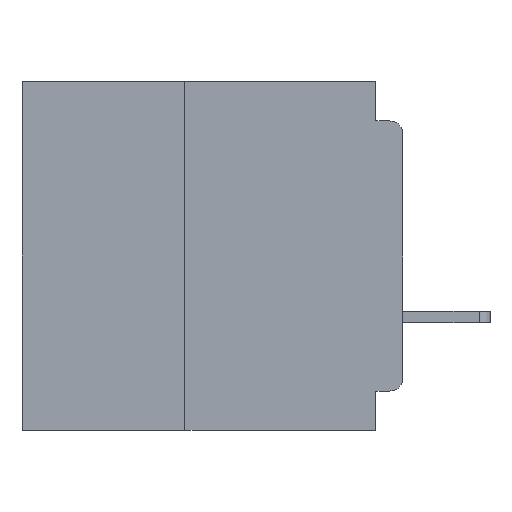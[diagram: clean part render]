
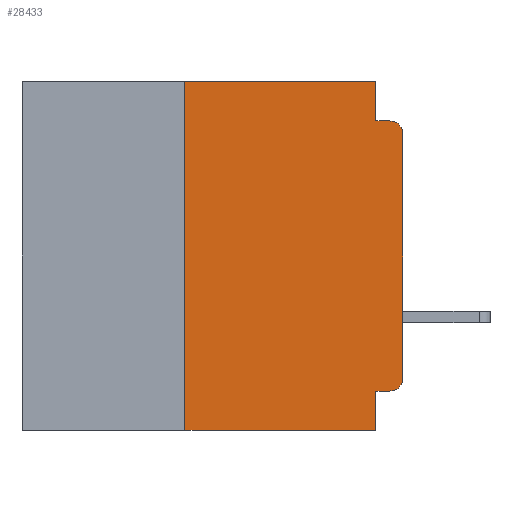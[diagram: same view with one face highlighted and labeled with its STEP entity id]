
A CAD part, left-side view. The second image highlights one B-rep face of the part: STEP entity #28433.
In plain terms, the highlighted planar face has unit normal (-1, 0, 0).
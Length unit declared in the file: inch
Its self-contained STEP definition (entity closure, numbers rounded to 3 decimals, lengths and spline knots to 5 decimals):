
#752 = CARTESIAN_POINT ( 'NONE',  ( 0., 0.031, -0.4 ) ) ;
#1406 = DIRECTION ( 'NONE',  ( 0., 0., -1. ) ) ;
#2109 = ORIENTED_EDGE ( 'NONE', *, *, #53110, .T. ) ;
#2112 = CARTESIAN_POINT ( 'NONE',  ( 0., 0.031, -0.4 ) ) ;
#2252 = FACE_OUTER_BOUND ( 'NONE', #7011, .T. ) ;
#3028 = ORIENTED_EDGE ( 'NONE', *, *, #6887, .F. ) ;
#6082 = VECTOR ( 'NONE', #15665, 39.37008 ) ;
#6200 = VECTOR ( 'NONE', #30947, 39.37008 ) ;
#6887 = EDGE_CURVE ( 'NONE', #15216, #43634, #40026, .T. ) ;
#7011 = EDGE_LOOP ( 'NONE', ( #31072, #17929, #53032, #22352, #19823, #24489, #22185, #44135, #3028, #2109 ) ) ;
#7617 = CARTESIAN_POINT ( 'NONE',  ( 0., 0.015, -0.045 ) ) ;
#7827 = CARTESIAN_POINT ( 'NONE',  ( 0., 0.25, 0. ) ) ;
#8480 = VERTEX_POINT ( 'NONE', #7617 ) ;
#9201 = CARTESIAN_POINT ( 'NONE',  ( 0., 0., 0. ) ) ;
#10609 = CARTESIAN_POINT ( 'NONE',  ( 0., 0., -0.06 ) ) ;
#11358 = CARTESIAN_POINT ( 'NONE',  ( 0., 0.437, -0.4 ) ) ;
#11630 = LINE ( 'NONE', #2112, #43968 ) ;
#11944 = CARTESIAN_POINT ( 'NONE',  ( 0., 0., -0.355 ) ) ;
#12194 = EDGE_CURVE ( 'NONE', #28208, #25364, #17548, .T. ) ;
#13304 = VECTOR ( 'NONE', #14707, 39.37008 ) ;
#13671 = EDGE_CURVE ( 'NONE', #28208, #19549, #39863, .T. ) ;
#14648 = LINE ( 'NONE', #31755, #13304 ) ;
#14707 = DIRECTION ( 'NONE',  ( 0., -1., 0. ) ) ;
#15216 = VERTEX_POINT ( 'NONE', #18132 ) ;
#15665 = DIRECTION ( 'NONE',  ( 0., -1., 0. ) ) ;
#17548 = LINE ( 'NONE', #18153, #6200 ) ;
#17929 = ORIENTED_EDGE ( 'NONE', *, *, #50631, .T. ) ;
#18132 = CARTESIAN_POINT ( 'NONE',  ( 0., 0.015, -0.355 ) ) ;
#18153 = CARTESIAN_POINT ( 'NONE',  ( 0., 0.25, -0.4 ) ) ;
#19419 = CARTESIAN_POINT ( 'NONE',  ( 0., 0.25, -0.4 ) ) ;
#19503 = VECTOR ( 'NONE', #51421, 39.37008 ) ;
#19549 = VERTEX_POINT ( 'NONE', #752 ) ;
#19823 = ORIENTED_EDGE ( 'NONE', *, *, #52072, .F. ) ;
#20182 = CARTESIAN_POINT ( 'NONE',  ( 0., 0., -0.045 ) ) ;
#20653 = DIRECTION ( 'NONE',  ( 0., 0., -1. ) ) ;
#21931 = CARTESIAN_POINT ( 'NONE',  ( 0., 0.015, -0.06 ) ) ;
#22185 = ORIENTED_EDGE ( 'NONE', *, *, #13671, .T. ) ;
#22352 = ORIENTED_EDGE ( 'NONE', *, *, #25996, .F. ) ;
#22805 = CIRCLE ( 'NONE', #50724, 0.015 ) ;
#23303 = DIRECTION ( 'NONE',  ( 0., 0., -1. ) ) ;
#23877 = LINE ( 'NONE', #20182, #35075 ) ;
#24489 = ORIENTED_EDGE ( 'NONE', *, *, #12194, .F. ) ;
#25311 = DIRECTION ( 'NONE',  ( 0., 0., -1. ) ) ;
#25364 = VERTEX_POINT ( 'NONE', #7827 ) ;
#25996 = EDGE_CURVE ( 'NONE', #26206, #37269, #47359, .T. ) ;
#26192 = DIRECTION ( 'NONE',  ( 0., 0., -1. ) ) ;
#26206 = VERTEX_POINT ( 'NONE', #51484 ) ;
#26882 = DIRECTION ( 'NONE',  ( -1., 0., 0. ) ) ;
#26962 = VERTEX_POINT ( 'NONE', #27810 ) ;
#27576 = VECTOR ( 'NONE', #54125, 39.37008 ) ;
#27722 = VECTOR ( 'NONE', #20653, 39.37008 ) ;
#27810 = CARTESIAN_POINT ( 'NONE',  ( 0., 0., -0.34 ) ) ;
#28208 = VERTEX_POINT ( 'NONE', #19419 ) ;
#28433 = ADVANCED_FACE ( 'NONE', ( #2252 ), #33412, .F. ) ;
#30947 = DIRECTION ( 'NONE',  ( 0., 0., 1. ) ) ;
#31072 = ORIENTED_EDGE ( 'NONE', *, *, #37814, .T. ) ;
#31755 = CARTESIAN_POINT ( 'NONE',  ( 0., 0.437, 0. ) ) ;
#32854 = CARTESIAN_POINT ( 'NONE',  ( 0., 0.031, -0.355 ) ) ;
#33412 = PLANE ( 'NONE',  #48881 ) ;
#35075 = VECTOR ( 'NONE', #53775, 39.37008 ) ;
#36321 = EDGE_CURVE ( 'NONE', #37269, #8480, #23877, .T. ) ;
#37269 = VERTEX_POINT ( 'NONE', #43424 ) ;
#37800 = CARTESIAN_POINT ( 'NONE',  ( 0., 0.437, 0. ) ) ;
#37814 = EDGE_CURVE ( 'NONE', #26962, #38660, #43195, .T. ) ;
#38660 = VERTEX_POINT ( 'NONE', #10609 ) ;
#39863 = LINE ( 'NONE', #11358, #6082 ) ;
#40026 = LINE ( 'NONE', #11944, #27576 ) ;
#43195 = LINE ( 'NONE', #9201, #19503 ) ;
#43424 = CARTESIAN_POINT ( 'NONE',  ( 0., 0.031, -0.045 ) ) ;
#43462 = EDGE_CURVE ( 'NONE', #43634, #19549, #11630, .T. ) ;
#43634 = VERTEX_POINT ( 'NONE', #32854 ) ;
#43968 = VECTOR ( 'NONE', #23303, 39.37008 ) ;
#44135 = ORIENTED_EDGE ( 'NONE', *, *, #43462, .F. ) ;
#45797 = CARTESIAN_POINT ( 'NONE',  ( 0., 0.031, 0. ) ) ;
#47359 = LINE ( 'NONE', #45797, #27722 ) ;
#48772 = CIRCLE ( 'NONE', #49754, 0.015 ) ;
#48881 = AXIS2_PLACEMENT_3D ( 'NONE', #37800, #50429, #25311 ) ;
#49754 = AXIS2_PLACEMENT_3D ( 'NONE', #51956, #26882, #1406 ) ;
#50429 = DIRECTION ( 'NONE',  ( 1., 0., 0. ) ) ;
#50631 = EDGE_CURVE ( 'NONE', #38660, #8480, #22805, .T. ) ;
#50724 = AXIS2_PLACEMENT_3D ( 'NONE', #21931, #51276, #26192 ) ;
#51276 = DIRECTION ( 'NONE',  ( -1., 0., 0. ) ) ;
#51421 = DIRECTION ( 'NONE',  ( 0., 0., 1. ) ) ;
#51484 = CARTESIAN_POINT ( 'NONE',  ( 0., 0.031, 0. ) ) ;
#51956 = CARTESIAN_POINT ( 'NONE',  ( 0., 0.015, -0.34 ) ) ;
#52072 = EDGE_CURVE ( 'NONE', #25364, #26206, #14648, .T. ) ;
#53032 = ORIENTED_EDGE ( 'NONE', *, *, #36321, .F. ) ;
#53110 = EDGE_CURVE ( 'NONE', #15216, #26962, #48772, .T. ) ;
#53775 = DIRECTION ( 'NONE',  ( 0., -1., 0. ) ) ;
#54125 = DIRECTION ( 'NONE',  ( 0., 1., 0. ) ) ;
